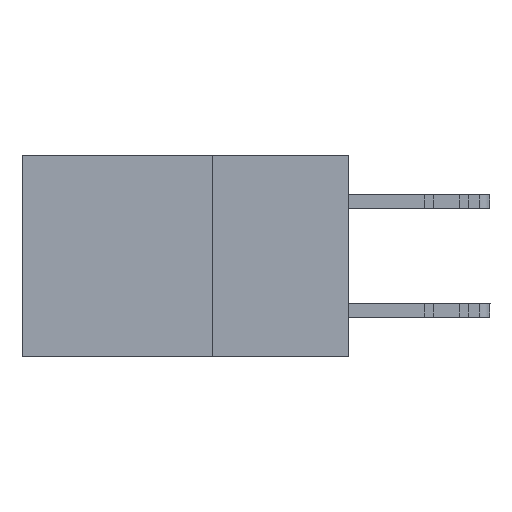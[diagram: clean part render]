
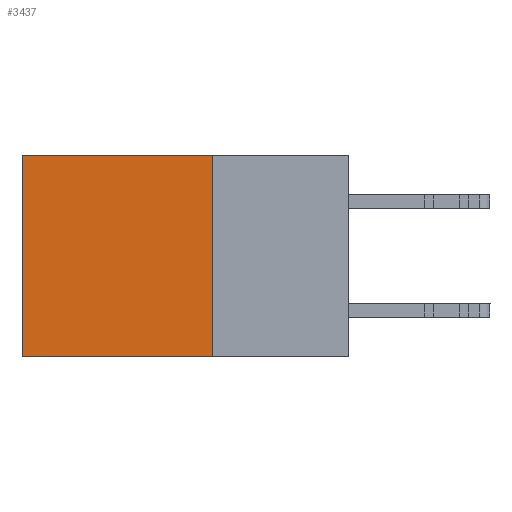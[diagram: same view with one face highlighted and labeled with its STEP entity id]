
A CAD part, left-side view. The second image highlights one B-rep face of the part: STEP entity #3437.
In plain terms, the highlighted planar face has unit normal (-1, 0, 0).
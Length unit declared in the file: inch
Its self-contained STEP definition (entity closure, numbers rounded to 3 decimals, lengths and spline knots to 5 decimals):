
#366 = CARTESIAN_POINT ( 'NONE',  ( 0.2615, 0.25, 0. ) ) ;
#805 = VERTEX_POINT ( 'NONE', #366 ) ;
#882 = AXIS2_PLACEMENT_3D ( 'NONE', #22525, #22481, #22216 ) ;
#1388 = EDGE_CURVE ( 'NONE', #12042, #24770, #2131, .T. ) ;
#2037 = EDGE_CURVE ( 'NONE', #805, #12042, #23867, .T. ) ;
#2131 = LINE ( 'NONE', #17309, #17371 ) ;
#2488 = DIRECTION ( 'NONE',  ( 0., 0., -1. ) ) ;
#3109 = VERTEX_POINT ( 'NONE', #6763 ) ;
#3283 = EDGE_CURVE ( 'NONE', #3109, #24770, #22085, .T. ) ;
#3311 = DIRECTION ( 'NONE',  ( 0., 1., 0. ) ) ;
#3437 = ADVANCED_FACE ( 'NONE', ( #8053 ), #25354, .F. ) ;
#3653 = ORIENTED_EDGE ( 'NONE', *, *, #3283, .T. ) ;
#6461 = VECTOR ( 'NONE', #8310, 39.37008 ) ;
#6763 = CARTESIAN_POINT ( 'NONE',  ( 0.2615, 0.6, 0. ) ) ;
#8053 = FACE_OUTER_BOUND ( 'NONE', #15264, .T. ) ;
#8310 = DIRECTION ( 'NONE',  ( 0., 0., -1. ) ) ;
#12042 = VERTEX_POINT ( 'NONE', #14276 ) ;
#13094 = CARTESIAN_POINT ( 'NONE',  ( 0.2615, 0.6, -0.37 ) ) ;
#13203 = ORIENTED_EDGE ( 'NONE', *, *, #2037, .F. ) ;
#13707 = CARTESIAN_POINT ( 'NONE',  ( 0.2615, 0.6, -0.37 ) ) ;
#14276 = CARTESIAN_POINT ( 'NONE',  ( 0.2615, 0.25, -0.37 ) ) ;
#15264 = EDGE_LOOP ( 'NONE', ( #3653, #16748, #13203, #24624 ) ) ;
#15539 = VECTOR ( 'NONE', #2488, 39.37008 ) ;
#16462 = VECTOR ( 'NONE', #3311, 39.37008 ) ;
#16748 = ORIENTED_EDGE ( 'NONE', *, *, #1388, .F. ) ;
#16946 = EDGE_CURVE ( 'NONE', #805, #3109, #17058, .T. ) ;
#17058 = LINE ( 'NONE', #17129, #16462 ) ;
#17129 = CARTESIAN_POINT ( 'NONE',  ( 0.2615, 0.25, 0. ) ) ;
#17309 = CARTESIAN_POINT ( 'NONE',  ( 0.2615, 0.25, -0.37 ) ) ;
#17371 = VECTOR ( 'NONE', #23378, 39.37008 ) ;
#22039 = CARTESIAN_POINT ( 'NONE',  ( 0.2615, 0.25, -0.37 ) ) ;
#22085 = LINE ( 'NONE', #13094, #6461 ) ;
#22216 = DIRECTION ( 'NONE',  ( 0., 0., -1. ) ) ;
#22481 = DIRECTION ( 'NONE',  ( 1., 0., 0. ) ) ;
#22525 = CARTESIAN_POINT ( 'NONE',  ( 0.2615, 0.25, -0.37 ) ) ;
#23378 = DIRECTION ( 'NONE',  ( 0., 1., 0. ) ) ;
#23867 = LINE ( 'NONE', #22039, #15539 ) ;
#24624 = ORIENTED_EDGE ( 'NONE', *, *, #16946, .T. ) ;
#24770 = VERTEX_POINT ( 'NONE', #13707 ) ;
#25354 = PLANE ( 'NONE',  #882 ) ;
